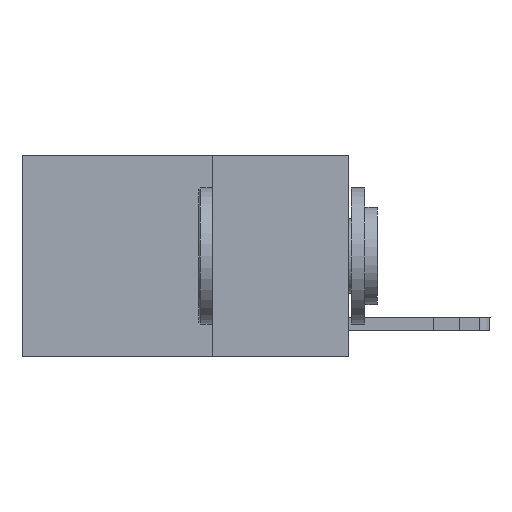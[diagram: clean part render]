
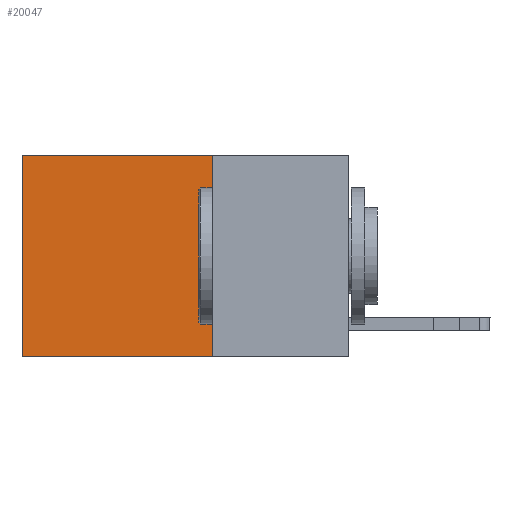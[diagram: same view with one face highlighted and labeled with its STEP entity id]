
A CAD part, left-side view. The second image highlights one B-rep face of the part: STEP entity #20047.
In plain terms, the highlighted planar face has unit normal (-1, 0, 0).
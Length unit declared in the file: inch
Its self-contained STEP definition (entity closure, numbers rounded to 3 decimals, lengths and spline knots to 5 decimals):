
#607 = ORIENTED_EDGE ( 'NONE', *, *, #23064, .F. ) ;
#835 = DIRECTION ( 'NONE',  ( 0., 1., 0. ) ) ;
#1026 = CARTESIAN_POINT ( 'NONE',  ( 0.2625, 0.6, -0.37 ) ) ;
#1207 = VERTEX_POINT ( 'NONE', #12408 ) ;
#1341 = ORIENTED_EDGE ( 'NONE', *, *, #13572, .T. ) ;
#1614 = CARTESIAN_POINT ( 'NONE',  ( 0.2625, 0.25, -0.37 ) ) ;
#2444 = VERTEX_POINT ( 'NONE', #25899 ) ;
#2936 = PLANE ( 'NONE',  #23588 ) ;
#3089 = VECTOR ( 'NONE', #835, 39.37008 ) ;
#4604 = CARTESIAN_POINT ( 'NONE',  ( 0.2625, 0.25, 0. ) ) ;
#5201 = ORIENTED_EDGE ( 'NONE', *, *, #18124, .T. ) ;
#6514 = DIRECTION ( 'NONE',  ( 0., 1., 0. ) ) ;
#8656 = LINE ( 'NONE', #9184, #20061 ) ;
#9006 = DIRECTION ( 'NONE',  ( 1., 0., 0. ) ) ;
#9184 = CARTESIAN_POINT ( 'NONE',  ( 0.2625, 0.25, 0. ) ) ;
#11148 = DIRECTION ( 'NONE',  ( 0., 0., -1. ) ) ;
#11322 = ORIENTED_EDGE ( 'NONE', *, *, #14517, .F. ) ;
#12408 = CARTESIAN_POINT ( 'NONE',  ( 0.2625, 0.25, 0. ) ) ;
#12740 = DIRECTION ( 'NONE',  ( 0., 0., -1. ) ) ;
#13572 = EDGE_CURVE ( 'NONE', #1207, #2444, #8656, .T. ) ;
#14517 = EDGE_CURVE ( 'NONE', #1207, #19800, #24669, .T. ) ;
#14826 = LINE ( 'NONE', #16975, #3089 ) ;
#14904 = EDGE_LOOP ( 'NONE', ( #5201, #607, #11322, #1341 ) ) ;
#15153 = CARTESIAN_POINT ( 'NONE',  ( 0.2625, 0.6, 0. ) ) ;
#15334 = DIRECTION ( 'NONE',  ( 0., 0., -1. ) ) ;
#15475 = VECTOR ( 'NONE', #15334, 39.37008 ) ;
#16975 = CARTESIAN_POINT ( 'NONE',  ( 0.2625, 0.25, -0.37 ) ) ;
#18124 = EDGE_CURVE ( 'NONE', #2444, #18318, #23507, .T. ) ;
#18318 = VERTEX_POINT ( 'NONE', #1026 ) ;
#19800 = VERTEX_POINT ( 'NONE', #1614 ) ;
#20047 = ADVANCED_FACE ( 'NONE', ( #23138 ), #2936, .F. ) ;
#20061 = VECTOR ( 'NONE', #6514, 39.37008 ) ;
#20987 = CARTESIAN_POINT ( 'NONE',  ( 0.2625, 0.25, 0. ) ) ;
#23064 = EDGE_CURVE ( 'NONE', #19800, #18318, #14826, .T. ) ;
#23138 = FACE_OUTER_BOUND ( 'NONE', #14904, .T. ) ;
#23507 = LINE ( 'NONE', #15153, #25299 ) ;
#23588 = AXIS2_PLACEMENT_3D ( 'NONE', #20987, #9006, #11148 ) ;
#24669 = LINE ( 'NONE', #4604, #15475 ) ;
#25299 = VECTOR ( 'NONE', #12740, 39.37008 ) ;
#25899 = CARTESIAN_POINT ( 'NONE',  ( 0.2625, 0.6, 0. ) ) ;
